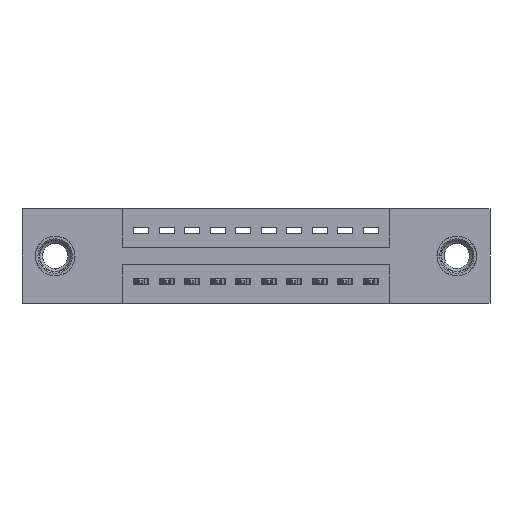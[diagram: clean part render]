
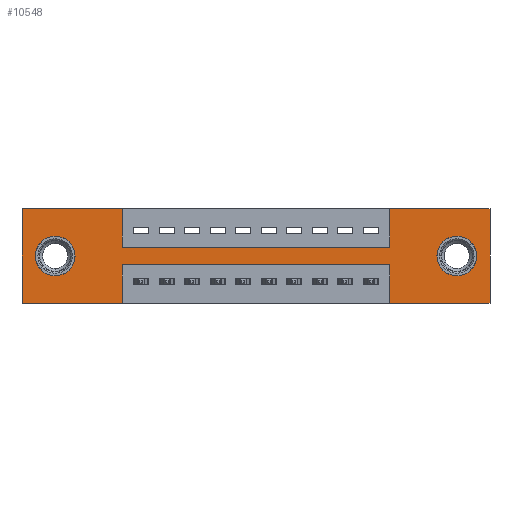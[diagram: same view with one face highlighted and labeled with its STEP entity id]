
A CAD part, front view. The second image highlights one B-rep face of the part: STEP entity #10548.
In plain terms, the highlighted planar face has unit normal (0, -1, 0).
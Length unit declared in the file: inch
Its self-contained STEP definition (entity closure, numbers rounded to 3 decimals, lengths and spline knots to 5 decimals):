
#9 = CARTESIAN_POINT ( 'NONE',  ( 0.13, 0., -0.263 ) ) ;
#44 = EDGE_CURVE ( 'NONE', #9258, #12856, #1756, .T. ) ;
#176 = VECTOR ( 'NONE', #8781, 39.37008 ) ;
#295 = ORIENTED_EDGE ( 'NONE', *, *, #4362, .F. ) ;
#561 = CARTESIAN_POINT ( 'NONE',  ( 1.705, 0., -0.263 ) ) ;
#574 = DIRECTION ( 'NONE',  ( -1., 0., 0. ) ) ;
#750 = CARTESIAN_POINT ( 'NONE',  ( 0., 0., -0.37 ) ) ;
#879 = EDGE_CURVE ( 'NONE', #1117, #8099, #3639, .T. ) ;
#996 = CARTESIAN_POINT ( 'NONE',  ( 1.705, 0., -0.185 ) ) ;
#1117 = VERTEX_POINT ( 'NONE', #1886 ) ;
#1273 = FACE_BOUND ( 'NONE', #4572, .T. ) ;
#1390 = ORIENTED_EDGE ( 'NONE', *, *, #1637, .F. ) ;
#1549 = VECTOR ( 'NONE', #12683, 39.37008 ) ;
#1637 = EDGE_CURVE ( 'NONE', #12856, #4728, #2816, .T. ) ;
#1667 = ORIENTED_EDGE ( 'NONE', *, *, #4916, .T. ) ;
#1741 = FACE_BOUND ( 'NONE', #9317, .T. ) ;
#1756 = LINE ( 'NONE', #12628, #12171 ) ;
#1762 = ORIENTED_EDGE ( 'NONE', *, *, #44, .F. ) ;
#1795 = ORIENTED_EDGE ( 'NONE', *, *, #879, .F. ) ;
#1886 = CARTESIAN_POINT ( 'NONE',  ( 1.4425, 0., 0. ) ) ;
#1973 = DIRECTION ( 'NONE',  ( 1., 0., 0. ) ) ;
#2116 = EDGE_CURVE ( 'NONE', #5904, #7507, #10824, .T. ) ;
#2226 = CARTESIAN_POINT ( 'NONE',  ( 0., 0., -0.37 ) ) ;
#2438 = VECTOR ( 'NONE', #3672, 39.37008 ) ;
#2580 = VERTEX_POINT ( 'NONE', #9 ) ;
#2695 = DIRECTION ( 'NONE',  ( 0., 1., 0. ) ) ;
#2750 = DIRECTION ( 'NONE',  ( 0., 1., 0. ) ) ;
#2816 = LINE ( 'NONE', #11772, #1549 ) ;
#2839 = DIRECTION ( 'NONE',  ( 0., 0., -1. ) ) ;
#2983 = VERTEX_POINT ( 'NONE', #6362 ) ;
#3084 = ORIENTED_EDGE ( 'NONE', *, *, #10560, .T. ) ;
#3087 = VERTEX_POINT ( 'NONE', #9762 ) ;
#3215 = ORIENTED_EDGE ( 'NONE', *, *, #2116, .F. ) ;
#3243 = CARTESIAN_POINT ( 'NONE',  ( 1.835, 0., -0.37 ) ) ;
#3300 = VERTEX_POINT ( 'NONE', #6567 ) ;
#3631 = AXIS2_PLACEMENT_3D ( 'NONE', #6966, #11940, #7140 ) ;
#3639 = LINE ( 'NONE', #6476, #6783 ) ;
#3672 = DIRECTION ( 'NONE',  ( 0., 0., -1. ) ) ;
#3733 = CARTESIAN_POINT ( 'NONE',  ( 1.705, 0., -0.185 ) ) ;
#3910 = CARTESIAN_POINT ( 'NONE',  ( 0.3925, 0., -0.15 ) ) ;
#4060 = ORIENTED_EDGE ( 'NONE', *, *, #4354, .F. ) ;
#4186 = AXIS2_PLACEMENT_3D ( 'NONE', #3733, #2750, #2839 ) ;
#4328 = VERTEX_POINT ( 'NONE', #3243 ) ;
#4354 = EDGE_CURVE ( 'NONE', #8099, #4328, #7485, .T. ) ;
#4362 = EDGE_CURVE ( 'NONE', #7507, #1117, #12808, .T. ) ;
#4484 = LINE ( 'NONE', #8909, #5427 ) ;
#4572 = EDGE_LOOP ( 'NONE', ( #1667, #3084 ) ) ;
#4620 = EDGE_CURVE ( 'NONE', #2983, #6869, #10464, .T. ) ;
#4624 = CARTESIAN_POINT ( 'NONE',  ( 0.3925, 0., -0.22 ) ) ;
#4728 = VERTEX_POINT ( 'NONE', #12146 ) ;
#4916 = EDGE_CURVE ( 'NONE', #3300, #6585, #7616, .T. ) ;
#5175 = CARTESIAN_POINT ( 'NONE',  ( 1.4425, 0., -0.37 ) ) ;
#5177 = CARTESIAN_POINT ( 'NONE',  ( 0.3925, 0., -0.22 ) ) ;
#5214 = CIRCLE ( 'NONE', #3631, 0.078 ) ;
#5427 = VECTOR ( 'NONE', #9980, 39.37008 ) ;
#5598 = CARTESIAN_POINT ( 'NONE',  ( 0., 0., -0.37 ) ) ;
#5634 = DIRECTION ( 'NONE',  ( -1., 0., 0. ) ) ;
#5672 = DIRECTION ( 'NONE',  ( 0., 0., -1. ) ) ;
#5849 = FACE_OUTER_BOUND ( 'NONE', #12884, .T. ) ;
#5904 = VERTEX_POINT ( 'NONE', #6956 ) ;
#6070 = DIRECTION ( 'NONE',  ( 0., 0., -1. ) ) ;
#6226 = CARTESIAN_POINT ( 'NONE',  ( 1.4425, 0., -0.37 ) ) ;
#6362 = CARTESIAN_POINT ( 'NONE',  ( 1.4425, 0., -0.22 ) ) ;
#6476 = CARTESIAN_POINT ( 'NONE',  ( 0., 0., 0. ) ) ;
#6567 = CARTESIAN_POINT ( 'NONE',  ( 1.705, 0., -0.107 ) ) ;
#6585 = VERTEX_POINT ( 'NONE', #561 ) ;
#6633 = CARTESIAN_POINT ( 'NONE',  ( 0.3925, 0., -0.37 ) ) ;
#6721 = DIRECTION ( 'NONE',  ( 0., 0., -1. ) ) ;
#6783 = VECTOR ( 'NONE', #7574, 39.37008 ) ;
#6869 = VERTEX_POINT ( 'NONE', #5177 ) ;
#6899 = CARTESIAN_POINT ( 'NONE',  ( 0.3925, 0., 0. ) ) ;
#6929 = CARTESIAN_POINT ( 'NONE',  ( 1.835, 0., 0. ) ) ;
#6945 = ORIENTED_EDGE ( 'NONE', *, *, #9151, .F. ) ;
#6956 = CARTESIAN_POINT ( 'NONE',  ( 0.3925, 0., -0.15 ) ) ;
#6966 = CARTESIAN_POINT ( 'NONE',  ( 0.13, 0., -0.185 ) ) ;
#7053 = ORIENTED_EDGE ( 'NONE', *, *, #7628, .T. ) ;
#7140 = DIRECTION ( 'NONE',  ( 0., 0., 1. ) ) ;
#7157 = EDGE_CURVE ( 'NONE', #9706, #2580, #11648, .T. ) ;
#7440 = VECTOR ( 'NONE', #11928, 39.37008 ) ;
#7485 = LINE ( 'NONE', #12850, #2438 ) ;
#7507 = VERTEX_POINT ( 'NONE', #8210 ) ;
#7574 = DIRECTION ( 'NONE',  ( 1., 0., 0. ) ) ;
#7616 = CIRCLE ( 'NONE', #10589, 0.078 ) ;
#7628 = EDGE_CURVE ( 'NONE', #2580, #9706, #5214, .T. ) ;
#7786 = VECTOR ( 'NONE', #10792, 39.37008 ) ;
#8099 = VERTEX_POINT ( 'NONE', #6929 ) ;
#8159 = CARTESIAN_POINT ( 'NONE',  ( 0.13, 0., -0.107 ) ) ;
#8210 = CARTESIAN_POINT ( 'NONE',  ( 1.4425, 0., -0.15 ) ) ;
#8250 = VERTEX_POINT ( 'NONE', #6226 ) ;
#8353 = ORIENTED_EDGE ( 'NONE', *, *, #12228, .F. ) ;
#8781 = DIRECTION ( 'NONE',  ( 0., 0., -1. ) ) ;
#8909 = CARTESIAN_POINT ( 'NONE',  ( 0., 0., 0. ) ) ;
#9057 = DIRECTION ( 'NONE',  ( 0., 1., 0. ) ) ;
#9151 = EDGE_CURVE ( 'NONE', #4728, #3087, #4484, .T. ) ;
#9258 = VERTEX_POINT ( 'NONE', #9468 ) ;
#9269 = DIRECTION ( 'NONE',  ( -1., 0., 0. ) ) ;
#9271 = ORIENTED_EDGE ( 'NONE', *, *, #10742, .F. ) ;
#9317 = EDGE_LOOP ( 'NONE', ( #11640, #7053 ) ) ;
#9468 = CARTESIAN_POINT ( 'NONE',  ( 0.3925, 0., -0.37 ) ) ;
#9617 = CARTESIAN_POINT ( 'NONE',  ( 0.13, 0., -0.185 ) ) ;
#9706 = VERTEX_POINT ( 'NONE', #8159 ) ;
#9753 = DIRECTION ( 'NONE',  ( 0., 0., 1. ) ) ;
#9762 = CARTESIAN_POINT ( 'NONE',  ( 0.3925, 0., 0. ) ) ;
#9980 = DIRECTION ( 'NONE',  ( 1., 0., 0. ) ) ;
#10222 = EDGE_CURVE ( 'NONE', #8250, #2983, #12767, .T. ) ;
#10262 = LINE ( 'NONE', #2226, #12301 ) ;
#10356 = ORIENTED_EDGE ( 'NONE', *, *, #10505, .F. ) ;
#10428 = LINE ( 'NONE', #6899, #176 ) ;
#10451 = ORIENTED_EDGE ( 'NONE', *, *, #4620, .F. ) ;
#10464 = LINE ( 'NONE', #4624, #12649 ) ;
#10502 = ORIENTED_EDGE ( 'NONE', *, *, #10222, .F. ) ;
#10505 = EDGE_CURVE ( 'NONE', #3087, #5904, #10428, .T. ) ;
#10548 = ADVANCED_FACE ( 'NONE', ( #1273, #1741, #5849 ), #12734, .T. ) ;
#10560 = EDGE_CURVE ( 'NONE', #6585, #3300, #11373, .T. ) ;
#10589 = AXIS2_PLACEMENT_3D ( 'NONE', #996, #9057, #6070 ) ;
#10742 = EDGE_CURVE ( 'NONE', #4328, #8250, #10262, .T. ) ;
#10761 = DIRECTION ( 'NONE',  ( 0., -1., 0. ) ) ;
#10792 = DIRECTION ( 'NONE',  ( 0., 0., 1. ) ) ;
#10824 = LINE ( 'NONE', #3910, #11618 ) ;
#11373 = CIRCLE ( 'NONE', #4186, 0.078 ) ;
#11467 = LINE ( 'NONE', #6633, #11950 ) ;
#11618 = VECTOR ( 'NONE', #1973, 39.37008 ) ;
#11640 = ORIENTED_EDGE ( 'NONE', *, *, #7157, .T. ) ;
#11648 = CIRCLE ( 'NONE', #11989, 0.078 ) ;
#11772 = CARTESIAN_POINT ( 'NONE',  ( 0., 0., 0. ) ) ;
#11928 = DIRECTION ( 'NONE',  ( 0., 0., 1. ) ) ;
#11940 = DIRECTION ( 'NONE',  ( 0., 1., 0. ) ) ;
#11950 = VECTOR ( 'NONE', #5672, 39.37008 ) ;
#11989 = AXIS2_PLACEMENT_3D ( 'NONE', #9617, #2695, #9753 ) ;
#12146 = CARTESIAN_POINT ( 'NONE',  ( 0., 0., 0. ) ) ;
#12171 = VECTOR ( 'NONE', #574, 39.37008 ) ;
#12228 = EDGE_CURVE ( 'NONE', #6869, #9258, #11467, .T. ) ;
#12301 = VECTOR ( 'NONE', #9269, 39.37008 ) ;
#12628 = CARTESIAN_POINT ( 'NONE',  ( 0., 0., -0.37 ) ) ;
#12649 = VECTOR ( 'NONE', #5634, 39.37008 ) ;
#12683 = DIRECTION ( 'NONE',  ( 0., 0., 1. ) ) ;
#12734 = PLANE ( 'NONE',  #13019 ) ;
#12767 = LINE ( 'NONE', #5175, #7440 ) ;
#12801 = CARTESIAN_POINT ( 'NONE',  ( 1.4425, 0., 0. ) ) ;
#12808 = LINE ( 'NONE', #12801, #7786 ) ;
#12850 = CARTESIAN_POINT ( 'NONE',  ( 1.835, 0., 0. ) ) ;
#12856 = VERTEX_POINT ( 'NONE', #5598 ) ;
#12884 = EDGE_LOOP ( 'NONE', ( #8353, #10451, #10502, #9271, #4060, #1795, #295, #3215, #10356, #6945, #1390, #1762 ) ) ;
#13019 = AXIS2_PLACEMENT_3D ( 'NONE', #750, #10761, #6721 ) ;
